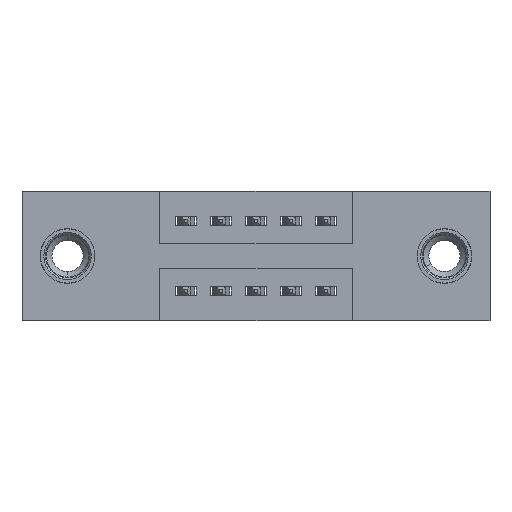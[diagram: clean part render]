
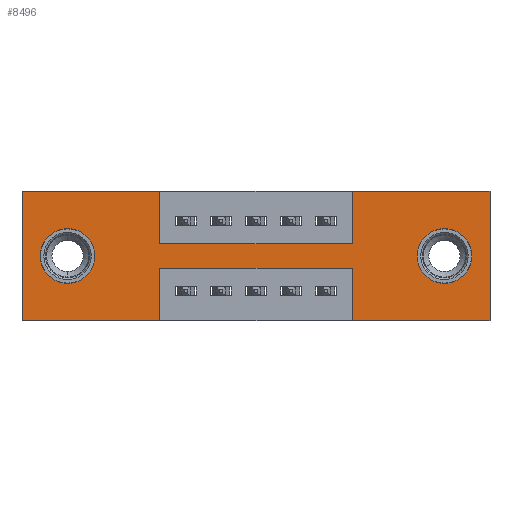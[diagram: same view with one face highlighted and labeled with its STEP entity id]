
A CAD part, front view. The second image highlights one B-rep face of the part: STEP entity #8496.
In plain terms, the highlighted planar face has unit normal (0, -1, 0).
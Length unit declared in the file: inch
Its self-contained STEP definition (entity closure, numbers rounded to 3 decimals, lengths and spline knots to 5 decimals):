
#96 = EDGE_CURVE ( 'NONE', #4066, #8494, #4402, .T. ) ;
#543 = VERTEX_POINT ( 'NONE', #9480 ) ;
#605 = DIRECTION ( 'NONE',  ( 1., 0., 0. ) ) ;
#642 = ORIENTED_EDGE ( 'NONE', *, *, #2477, .T. ) ;
#650 = CARTESIAN_POINT ( 'NONE',  ( 0.3925, 0., 0. ) ) ;
#676 = CARTESIAN_POINT ( 'NONE',  ( 0.13, 0., -0.185 ) ) ;
#805 = EDGE_CURVE ( 'NONE', #1485, #965, #5887, .T. ) ;
#901 = VERTEX_POINT ( 'NONE', #8072 ) ;
#965 = VERTEX_POINT ( 'NONE', #4770 ) ;
#1021 = CARTESIAN_POINT ( 'NONE',  ( 0.3925, 0., -0.15 ) ) ;
#1115 = DIRECTION ( 'NONE',  ( 1., 0., 0. ) ) ;
#1139 = EDGE_CURVE ( 'NONE', #6125, #8276, #9889, .T. ) ;
#1224 = CARTESIAN_POINT ( 'NONE',  ( 0.9425, 0., -0.37 ) ) ;
#1239 = ORIENTED_EDGE ( 'NONE', *, *, #5528, .F. ) ;
#1349 = DIRECTION ( 'NONE',  ( -1., 0., 0. ) ) ;
#1367 = ORIENTED_EDGE ( 'NONE', *, *, #7642, .F. ) ;
#1427 = VECTOR ( 'NONE', #1492, 39.37008 ) ;
#1451 = DIRECTION ( 'NONE',  ( 0., 0., 1. ) ) ;
#1485 = VERTEX_POINT ( 'NONE', #7051 ) ;
#1492 = DIRECTION ( 'NONE',  ( 0., 0., -1. ) ) ;
#1538 = DIRECTION ( 'NONE',  ( 0., 1., 0. ) ) ;
#1555 = CARTESIAN_POINT ( 'NONE',  ( 0., 0., -0.37 ) ) ;
#1690 = VECTOR ( 'NONE', #4485, 39.37008 ) ;
#1791 = EDGE_CURVE ( 'NONE', #8269, #2021, #3755, .T. ) ;
#1826 = VECTOR ( 'NONE', #10106, 39.37008 ) ;
#1956 = CIRCLE ( 'NONE', #8327, 0.078 ) ;
#2021 = VERTEX_POINT ( 'NONE', #650 ) ;
#2077 = AXIS2_PLACEMENT_3D ( 'NONE', #6228, #6999, #2291 ) ;
#2081 = VECTOR ( 'NONE', #7263, 39.37008 ) ;
#2102 = CARTESIAN_POINT ( 'NONE',  ( 0.9425, 0., 0. ) ) ;
#2291 = DIRECTION ( 'NONE',  ( 0., 0., -1. ) ) ;
#2477 = EDGE_CURVE ( 'NONE', #901, #8396, #8109, .T. ) ;
#2572 = VERTEX_POINT ( 'NONE', #1555 ) ;
#2762 = CARTESIAN_POINT ( 'NONE',  ( 0., 0., 0. ) ) ;
#2766 = CARTESIAN_POINT ( 'NONE',  ( 0.3925, 0., -0.22 ) ) ;
#2851 = CARTESIAN_POINT ( 'NONE',  ( 1.205, 0., -0.185 ) ) ;
#3107 = ORIENTED_EDGE ( 'NONE', *, *, #1791, .F. ) ;
#3174 = VECTOR ( 'NONE', #605, 39.37008 ) ;
#3226 = EDGE_LOOP ( 'NONE', ( #6670, #642 ) ) ;
#3345 = ORIENTED_EDGE ( 'NONE', *, *, #8399, .F. ) ;
#3459 = CARTESIAN_POINT ( 'NONE',  ( 0., 0., 0. ) ) ;
#3500 = DIRECTION ( 'NONE',  ( 0., 1., 0. ) ) ;
#3516 = LINE ( 'NONE', #10080, #1427 ) ;
#3588 = CARTESIAN_POINT ( 'NONE',  ( 0.9425, 0., -0.22 ) ) ;
#3634 = DIRECTION ( 'NONE',  ( 0., 0., -1. ) ) ;
#3647 = VECTOR ( 'NONE', #6856, 39.37008 ) ;
#3692 = CARTESIAN_POINT ( 'NONE',  ( 0.3925, 0., -0.37 ) ) ;
#3712 = LINE ( 'NONE', #8433, #7632 ) ;
#3718 = AXIS2_PLACEMENT_3D ( 'NONE', #8212, #3500, #9003 ) ;
#3755 = LINE ( 'NONE', #3459, #9745 ) ;
#3901 = LINE ( 'NONE', #10132, #9899 ) ;
#4066 = VERTEX_POINT ( 'NONE', #3588 ) ;
#4154 = LINE ( 'NONE', #9590, #2081 ) ;
#4221 = EDGE_CURVE ( 'NONE', #965, #9605, #7331, .T. ) ;
#4402 = LINE ( 'NONE', #2766, #1826 ) ;
#4485 = DIRECTION ( 'NONE',  ( 0., 0., 1. ) ) ;
#4571 = ORIENTED_EDGE ( 'NONE', *, *, #5742, .T. ) ;
#4770 = CARTESIAN_POINT ( 'NONE',  ( 0.9425, 0., 0. ) ) ;
#4827 = EDGE_CURVE ( 'NONE', #9605, #6125, #3516, .T. ) ;
#5047 = ORIENTED_EDGE ( 'NONE', *, *, #9359, .F. ) ;
#5223 = VERTEX_POINT ( 'NONE', #3692 ) ;
#5271 = CARTESIAN_POINT ( 'NONE',  ( 0.3925, 0., 0. ) ) ;
#5421 = PLANE ( 'NONE',  #2077 ) ;
#5528 = EDGE_CURVE ( 'NONE', #2572, #8269, #7686, .T. ) ;
#5641 = CARTESIAN_POINT ( 'NONE',  ( 0., 0., -0.37 ) ) ;
#5650 = AXIS2_PLACEMENT_3D ( 'NONE', #6277, #1538, #7049 ) ;
#5742 = EDGE_CURVE ( 'NONE', #7258, #543, #6014, .T. ) ;
#5792 = FACE_BOUND ( 'NONE', #3226, .T. ) ;
#5883 = VECTOR ( 'NONE', #7148, 39.37008 ) ;
#5887 = LINE ( 'NONE', #2102, #1690 ) ;
#5956 = CARTESIAN_POINT ( 'NONE',  ( 0.9425, 0., -0.37 ) ) ;
#5968 = DIRECTION ( 'NONE',  ( 0., 0., 1. ) ) ;
#6014 = CIRCLE ( 'NONE', #3718, 0.078 ) ;
#6025 = CARTESIAN_POINT ( 'NONE',  ( 1.205, 0., -0.263 ) ) ;
#6082 = EDGE_CURVE ( 'NONE', #8396, #901, #7439, .T. ) ;
#6125 = VERTEX_POINT ( 'NONE', #10123 ) ;
#6204 = DIRECTION ( 'NONE',  ( 0., 1., 0. ) ) ;
#6228 = CARTESIAN_POINT ( 'NONE',  ( 0., 0., -0.37 ) ) ;
#6277 = CARTESIAN_POINT ( 'NONE',  ( 0.13, 0., -0.185 ) ) ;
#6301 = DIRECTION ( 'NONE',  ( 1., 0., 0. ) ) ;
#6413 = AXIS2_PLACEMENT_3D ( 'NONE', #676, #6204, #1451 ) ;
#6426 = ORIENTED_EDGE ( 'NONE', *, *, #9674, .T. ) ;
#6443 = VECTOR ( 'NONE', #5968, 39.37008 ) ;
#6549 = ORIENTED_EDGE ( 'NONE', *, *, #805, .F. ) ;
#6670 = ORIENTED_EDGE ( 'NONE', *, *, #6082, .T. ) ;
#6851 = CARTESIAN_POINT ( 'NONE',  ( 0.13, 0., -0.107 ) ) ;
#6856 = DIRECTION ( 'NONE',  ( -1., 0., 0. ) ) ;
#6924 = CARTESIAN_POINT ( 'NONE',  ( 0.3925, 0., -0.22 ) ) ;
#6999 = DIRECTION ( 'NONE',  ( 0., -1., 0. ) ) ;
#7049 = DIRECTION ( 'NONE',  ( 0., 0., 1. ) ) ;
#7051 = CARTESIAN_POINT ( 'NONE',  ( 0.9425, 0., -0.15 ) ) ;
#7148 = DIRECTION ( 'NONE',  ( 0., 0., 1. ) ) ;
#7258 = VERTEX_POINT ( 'NONE', #6025 ) ;
#7263 = DIRECTION ( 'NONE',  ( 0., 0., -1. ) ) ;
#7331 = LINE ( 'NONE', #9220, #3174 ) ;
#7439 = CIRCLE ( 'NONE', #5650, 0.078 ) ;
#7492 = VERTEX_POINT ( 'NONE', #1021 ) ;
#7632 = VECTOR ( 'NONE', #1349, 39.37008 ) ;
#7642 = EDGE_CURVE ( 'NONE', #8276, #4066, #8527, .T. ) ;
#7686 = LINE ( 'NONE', #7954, #5883 ) ;
#7837 = FACE_BOUND ( 'NONE', #9873, .T. ) ;
#7858 = LINE ( 'NONE', #5271, #9953 ) ;
#7954 = CARTESIAN_POINT ( 'NONE',  ( 0., 0., 0. ) ) ;
#8072 = CARTESIAN_POINT ( 'NONE',  ( 0.13, 0., -0.263 ) ) ;
#8109 = CIRCLE ( 'NONE', #6413, 0.078 ) ;
#8111 = EDGE_LOOP ( 'NONE', ( #5047, #9468, #1367, #9703, #9949, #8120, #6549, #8629, #8876, #3107, #1239, #3345 ) ) ;
#8120 = ORIENTED_EDGE ( 'NONE', *, *, #4221, .F. ) ;
#8212 = CARTESIAN_POINT ( 'NONE',  ( 1.205, 0., -0.185 ) ) ;
#8269 = VERTEX_POINT ( 'NONE', #2762 ) ;
#8276 = VERTEX_POINT ( 'NONE', #5956 ) ;
#8327 = AXIS2_PLACEMENT_3D ( 'NONE', #2851, #8342, #3634 ) ;
#8342 = DIRECTION ( 'NONE',  ( 0., 1., 0. ) ) ;
#8386 = EDGE_CURVE ( 'NONE', #2021, #7492, #7858, .T. ) ;
#8396 = VERTEX_POINT ( 'NONE', #6851 ) ;
#8399 = EDGE_CURVE ( 'NONE', #5223, #2572, #3712, .T. ) ;
#8433 = CARTESIAN_POINT ( 'NONE',  ( 0., 0., -0.37 ) ) ;
#8494 = VERTEX_POINT ( 'NONE', #6924 ) ;
#8496 = ADVANCED_FACE ( 'NONE', ( #7837, #5792, #9929 ), #5421, .T. ) ;
#8527 = LINE ( 'NONE', #1224, #6443 ) ;
#8629 = ORIENTED_EDGE ( 'NONE', *, *, #9933, .F. ) ;
#8876 = ORIENTED_EDGE ( 'NONE', *, *, #8386, .F. ) ;
#9003 = DIRECTION ( 'NONE',  ( 0., 0., -1. ) ) ;
#9180 = DIRECTION ( 'NONE',  ( 0., 0., -1. ) ) ;
#9220 = CARTESIAN_POINT ( 'NONE',  ( 0., 0., 0. ) ) ;
#9359 = EDGE_CURVE ( 'NONE', #8494, #5223, #4154, .T. ) ;
#9468 = ORIENTED_EDGE ( 'NONE', *, *, #96, .F. ) ;
#9480 = CARTESIAN_POINT ( 'NONE',  ( 1.205, 0., -0.107 ) ) ;
#9590 = CARTESIAN_POINT ( 'NONE',  ( 0.3925, 0., -0.37 ) ) ;
#9605 = VERTEX_POINT ( 'NONE', #9824 ) ;
#9674 = EDGE_CURVE ( 'NONE', #543, #7258, #1956, .T. ) ;
#9703 = ORIENTED_EDGE ( 'NONE', *, *, #1139, .F. ) ;
#9745 = VECTOR ( 'NONE', #1115, 39.37008 ) ;
#9824 = CARTESIAN_POINT ( 'NONE',  ( 1.335, 0., 0. ) ) ;
#9873 = EDGE_LOOP ( 'NONE', ( #6426, #4571 ) ) ;
#9889 = LINE ( 'NONE', #5641, #3647 ) ;
#9899 = VECTOR ( 'NONE', #6301, 39.37008 ) ;
#9929 = FACE_OUTER_BOUND ( 'NONE', #8111, .T. ) ;
#9933 = EDGE_CURVE ( 'NONE', #7492, #1485, #3901, .T. ) ;
#9949 = ORIENTED_EDGE ( 'NONE', *, *, #4827, .F. ) ;
#9953 = VECTOR ( 'NONE', #9180, 39.37008 ) ;
#10080 = CARTESIAN_POINT ( 'NONE',  ( 1.335, 0., 0. ) ) ;
#10106 = DIRECTION ( 'NONE',  ( -1., 0., 0. ) ) ;
#10123 = CARTESIAN_POINT ( 'NONE',  ( 1.335, 0., -0.37 ) ) ;
#10132 = CARTESIAN_POINT ( 'NONE',  ( 0.3925, 0., -0.15 ) ) ;
